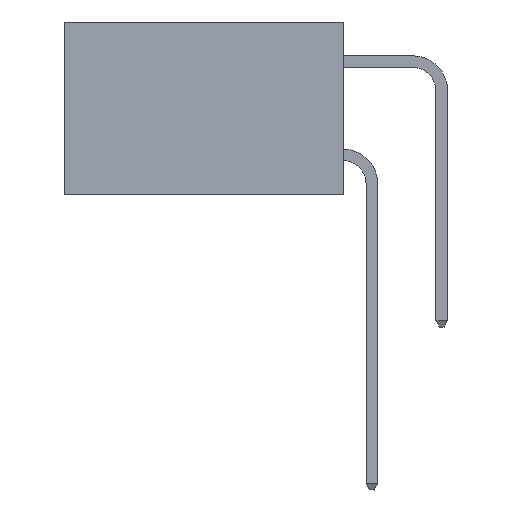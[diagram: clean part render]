
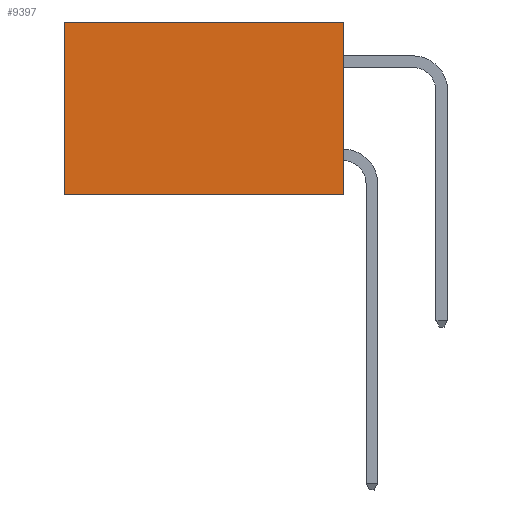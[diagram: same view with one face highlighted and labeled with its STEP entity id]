
A CAD part, left-side view. The second image highlights one B-rep face of the part: STEP entity #9397.
In plain terms, the highlighted planar face has unit normal (-1, 0, 0).
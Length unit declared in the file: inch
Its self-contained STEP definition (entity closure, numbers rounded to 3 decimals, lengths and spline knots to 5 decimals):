
#104 = AXIS2_PLACEMENT_3D ( 'NONE', #19107, #8289, #13169 ) ;
#1575 = VERTEX_POINT ( 'NONE', #10686 ) ;
#1843 = CARTESIAN_POINT ( 'NONE',  ( 0.2615, 0., 0. ) ) ;
#2244 = CARTESIAN_POINT ( 'NONE',  ( 0.2615, 0.6, 0. ) ) ;
#4468 = LINE ( 'NONE', #10749, #15666 ) ;
#4682 = EDGE_CURVE ( 'NONE', #13676, #19057, #13496, .T. ) ;
#5108 = VECTOR ( 'NONE', #15066, 39.37008 ) ;
#6658 = PLANE ( 'NONE',  #104 ) ;
#6887 = LINE ( 'NONE', #13197, #19903 ) ;
#7990 = FACE_OUTER_BOUND ( 'NONE', #14215, .T. ) ;
#8289 = DIRECTION ( 'NONE',  ( 1., 0., 0. ) ) ;
#8529 = DIRECTION ( 'NONE',  ( 0., 0., -1. ) ) ;
#8768 = VECTOR ( 'NONE', #12268, 39.37008 ) ;
#9397 = ADVANCED_FACE ( 'NONE', ( #7990 ), #6658, .F. ) ;
#10686 = CARTESIAN_POINT ( 'NONE',  ( 0.2615, 0.6, -0.37 ) ) ;
#10749 = CARTESIAN_POINT ( 'NONE',  ( 0.2615, 0., 0. ) ) ;
#11623 = CARTESIAN_POINT ( 'NONE',  ( 0.2615, 0., -0.37 ) ) ;
#12268 = DIRECTION ( 'NONE',  ( 0., 1., 0. ) ) ;
#13169 = DIRECTION ( 'NONE',  ( 0., 0., -1. ) ) ;
#13197 = CARTESIAN_POINT ( 'NONE',  ( 0.2615, 0.6, -0.37 ) ) ;
#13496 = LINE ( 'NONE', #11623, #5108 ) ;
#13676 = VERTEX_POINT ( 'NONE', #1843 ) ;
#13767 = VERTEX_POINT ( 'NONE', #2244 ) ;
#14155 = ORIENTED_EDGE ( 'NONE', *, *, #4682, .F. ) ;
#14215 = EDGE_LOOP ( 'NONE', ( #18584, #15703, #14155, #19434 ) ) ;
#15066 = DIRECTION ( 'NONE',  ( 0., 0., -1. ) ) ;
#15666 = VECTOR ( 'NONE', #17023, 39.37008 ) ;
#15703 = ORIENTED_EDGE ( 'NONE', *, *, #20276, .F. ) ;
#17023 = DIRECTION ( 'NONE',  ( 0., 1., 0. ) ) ;
#18187 = EDGE_CURVE ( 'NONE', #13676, #13767, #4468, .T. ) ;
#18584 = ORIENTED_EDGE ( 'NONE', *, *, #18911, .T. ) ;
#18911 = EDGE_CURVE ( 'NONE', #13767, #1575, #6887, .T. ) ;
#19057 = VERTEX_POINT ( 'NONE', #20157 ) ;
#19107 = CARTESIAN_POINT ( 'NONE',  ( 0.2615, 0., -0.37 ) ) ;
#19434 = ORIENTED_EDGE ( 'NONE', *, *, #18187, .T. ) ;
#19903 = VECTOR ( 'NONE', #8529, 39.37008 ) ;
#20157 = CARTESIAN_POINT ( 'NONE',  ( 0.2615, 0., -0.37 ) ) ;
#20161 = CARTESIAN_POINT ( 'NONE',  ( 0.2615, 0., -0.37 ) ) ;
#20262 = LINE ( 'NONE', #20161, #8768 ) ;
#20276 = EDGE_CURVE ( 'NONE', #19057, #1575, #20262, .T. ) ;
